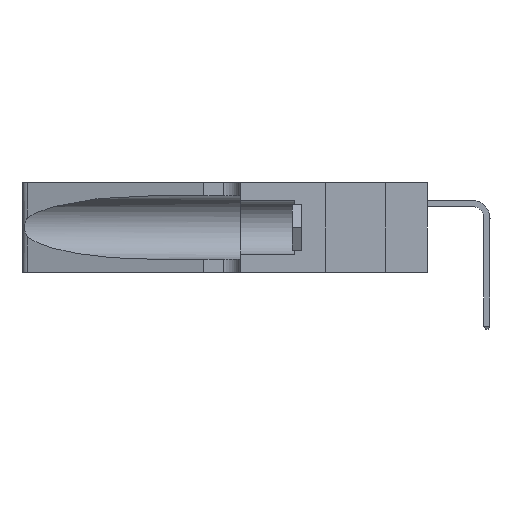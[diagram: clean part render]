
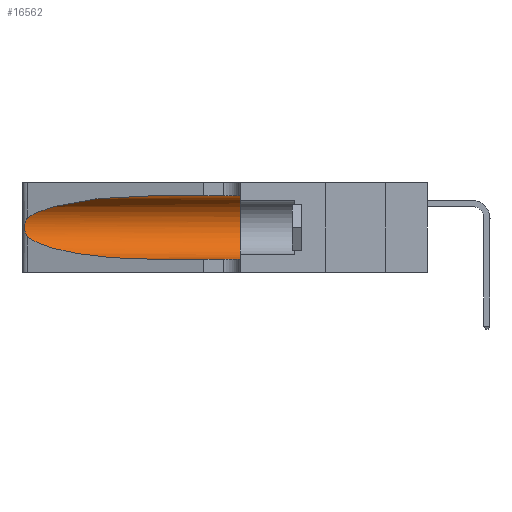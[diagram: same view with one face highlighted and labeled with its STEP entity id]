
A CAD part, left-side view. The second image highlights one B-rep face of the part: STEP entity #16562.
In plain terms, the highlighted cylindrical face has radius 3.308 mm (diameter 6.617 mm), a partial arc.
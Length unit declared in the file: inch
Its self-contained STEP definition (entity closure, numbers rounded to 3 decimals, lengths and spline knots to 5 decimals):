
#302 = ORIENTED_EDGE ( 'NONE', *, *, #26573, .T. ) ;
#671 = CARTESIAN_POINT ( 'NONE',  ( 0.25487, 1.22718, 0.14631 ) ) ;
#2597 = CARTESIAN_POINT ( 'NONE',  ( 0.25789, 1.23486, 0.15765 ) ) ;
#2893 = CARTESIAN_POINT ( 'NONE',  ( 0.1305, 1.61858, 0.05475 ) ) ;
#3138 = ORIENTED_EDGE ( 'NONE', *, *, #42239, .T. ) ;
#3344 = VERTEX_POINT ( 'NONE', #34396 ) ;
#3776 = VERTEX_POINT ( 'NONE', #13553 ) ;
#3834 = CARTESIAN_POINT ( 'NONE',  ( 0.1305, 0.72297, 0.31525 ) ) ;
#5797 = CARTESIAN_POINT ( 'NONE',  ( 0.25555, 1.22994, 0.2215 ) ) ;
#5943 = CARTESIAN_POINT ( 'NONE',  ( 0.25555, 1.22993, 0.14849 ) ) ;
#7239 = CARTESIAN_POINT ( 'NONE',  ( 0.25487, 1.22718, 0.14631 ) ) ;
#7544 = LINE ( 'NONE', #11586, #25005 ) ;
#9405 = CARTESIAN_POINT ( 'NONE',  ( 0.1305, 0.72297, 0.05475 ) ) ;
#9570 = VERTEX_POINT ( 'NONE', #9405 ) ;
#9579 =( BOUNDED_CURVE ( )  B_SPLINE_CURVE ( 3, ( #3834, #30153, #13754, #36730 ),
 .UNSPECIFIED., .F., .F. ) 
 B_SPLINE_CURVE_WITH_KNOTS ( ( 4, 4 ),
 ( 1.5708, 2.84003 ),
 .UNSPECIFIED. ) 
 CURVE ( )  GEOMETRIC_REPRESENTATION_ITEM ( )  RATIONAL_B_SPLINE_CURVE ( ( 1., 0.87, 0.87, 1. ) ) 
 REPRESENTATION_ITEM ( '' )  );
#9707 = DIRECTION ( 'NONE',  ( 0., -1., 0. ) ) ;
#10132 = ORIENTED_EDGE ( 'NONE', *, *, #27444, .F. ) ;
#10673 = CARTESIAN_POINT ( 'NONE',  ( 0.1305, 0.72297, 0.05475 ) ) ;
#11586 = CARTESIAN_POINT ( 'NONE',  ( 0.1305, 1.61858, 0.31525 ) ) ;
#12404 = CARTESIAN_POINT ( 'NONE',  ( 0.25787, 1.23484, 0.2124 ) ) ;
#12411 = LINE ( 'NONE', #2893, #38629 ) ;
#13399 = CARTESIAN_POINT ( 'NONE',  ( 0.1305, 1.61858, 0.185 ) ) ;
#13553 = CARTESIAN_POINT ( 'NONE',  ( 0.1305, 0.35, 0.31525 ) ) ;
#13754 = CARTESIAN_POINT ( 'NONE',  ( 0.2373, 1.15595, 0.28018 ) ) ;
#14033 = CARTESIAN_POINT ( 'NONE',  ( 0.1305, 0.72297, 0.31525 ) ) ;
#14101 = VERTEX_POINT ( 'NONE', #26527 ) ;
#14123 = AXIS2_PLACEMENT_3D ( 'NONE', #14925, #37875, #18237 ) ;
#14925 = CARTESIAN_POINT ( 'NONE',  ( 0.1305, 0.35, 0.185 ) ) ;
#15762 = CARTESIAN_POINT ( 'NONE',  ( 0.26018, 1.23835, 0.19895 ) ) ;
#16562 = ADVANCED_FACE ( 'NONE', ( #36401 ), #35370, .F. ) ;
#18237 = DIRECTION ( 'NONE',  ( 0., 0., 1. ) ) ;
#18922 = CARTESIAN_POINT ( 'NONE',  ( 0.25487, 1.22718, 0.22369 ) ) ;
#19068 = CARTESIAN_POINT ( 'NONE',  ( 0.26075, 1.23896, 0.178 ) ) ;
#20401 =( BOUNDED_CURVE ( )  B_SPLINE_CURVE ( 3, ( #671, #20467, #30360, #10673 ),
 .UNSPECIFIED., .F., .F. ) 
 B_SPLINE_CURVE_WITH_KNOTS ( ( 4, 4 ),
 ( 3.44316, 4.71239 ),
 .UNSPECIFIED. ) 
 CURVE ( )  GEOMETRIC_REPRESENTATION_ITEM ( )  RATIONAL_B_SPLINE_CURVE ( ( 1., 0.87, 0.87, 1. ) ) 
 REPRESENTATION_ITEM ( '' )  );
#20467 = CARTESIAN_POINT ( 'NONE',  ( 0.2373, 1.15595, 0.08982 ) ) ;
#21877 = EDGE_LOOP ( 'NONE', ( #26416, #3138, #302, #33444, #10132, #28252 ) ) ;
#22336 = CARTESIAN_POINT ( 'NONE',  ( 0.25856, 1.23593, 0.16098 ) ) ;
#24766 = VERTEX_POINT ( 'NONE', #7239 ) ;
#25005 = VECTOR ( 'NONE', #34553, 39.37008 ) ;
#25630 = CARTESIAN_POINT ( 'NONE',  ( 0.25639, 1.23186, 0.15144 ) ) ;
#26416 = ORIENTED_EDGE ( 'NONE', *, *, #38683, .T. ) ;
#26527 = CARTESIAN_POINT ( 'NONE',  ( 0.1305, 0.35, 0.05475 ) ) ;
#26573 = EDGE_CURVE ( 'NONE', #24766, #9570, #20401, .T. ) ;
#27444 = EDGE_CURVE ( 'NONE', #3776, #14101, #27899, .T. ) ;
#27899 = CIRCLE ( 'NONE', #14123, 0.13025 ) ;
#28252 = ORIENTED_EDGE ( 'NONE', *, *, #31370, .F. ) ;
#28954 = CARTESIAN_POINT ( 'NONE',  ( 0.25487, 1.22718, 0.14631 ) ) ;
#30127 = AXIS2_PLACEMENT_3D ( 'NONE', #13399, #36378, #33056 ) ;
#30153 = CARTESIAN_POINT ( 'NONE',  ( 0.18966, 0.96281, 0.31525 ) ) ;
#30360 = CARTESIAN_POINT ( 'NONE',  ( 0.18966, 0.96281, 0.05475 ) ) ;
#31370 = EDGE_CURVE ( 'NONE', #32337, #3776, #7544, .T. ) ;
#31402 = B_SPLINE_CURVE_WITH_KNOTS ( 'NONE', 3,
 ( #18922, #5797, #32108, #12404, #35398, #15762, #38693, #19068, #41968, #22336, #2597, #25630, #5943, #28954 ),
 .UNSPECIFIED., .F., .F.,
 ( 4, 2, 2, 2, 2, 2, 4 ),
 ( 0., 0.00027, 0.00053, 0.00107, 0.0016, 0.00187, 0.00214 ),
 .UNSPECIFIED. ) ;
#32108 = CARTESIAN_POINT ( 'NONE',  ( 0.25639, 1.23184, 0.21858 ) ) ;
#32337 = VERTEX_POINT ( 'NONE', #14033 ) ;
#33056 = DIRECTION ( 'NONE',  ( 0., 0., -1. ) ) ;
#33444 = ORIENTED_EDGE ( 'NONE', *, *, #37336, .T. ) ;
#34396 = CARTESIAN_POINT ( 'NONE',  ( 0.25487, 1.22718, 0.22369 ) ) ;
#34553 = DIRECTION ( 'NONE',  ( 0., -1., 0. ) ) ;
#35370 = CYLINDRICAL_SURFACE ( 'NONE', #30127, 0.13025 ) ;
#35398 = CARTESIAN_POINT ( 'NONE',  ( 0.25854, 1.2359, 0.20912 ) ) ;
#36378 = DIRECTION ( 'NONE',  ( 0., -1., 0. ) ) ;
#36401 = FACE_OUTER_BOUND ( 'NONE', #21877, .T. ) ;
#36730 = CARTESIAN_POINT ( 'NONE',  ( 0.25487, 1.22718, 0.22369 ) ) ;
#37336 = EDGE_CURVE ( 'NONE', #9570, #14101, #12411, .T. ) ;
#37875 = DIRECTION ( 'NONE',  ( 0., 1., 0. ) ) ;
#38629 = VECTOR ( 'NONE', #9707, 39.37008 ) ;
#38683 = EDGE_CURVE ( 'NONE', #32337, #3344, #9579, .T. ) ;
#38693 = CARTESIAN_POINT ( 'NONE',  ( 0.26075, 1.23896, 0.19203 ) ) ;
#41968 = CARTESIAN_POINT ( 'NONE',  ( 0.26017, 1.23833, 0.17102 ) ) ;
#42239 = EDGE_CURVE ( 'NONE', #3344, #24766, #31402, .T. ) ;
